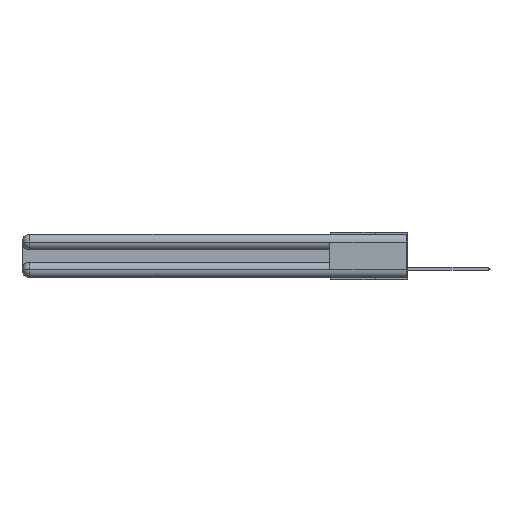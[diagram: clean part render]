
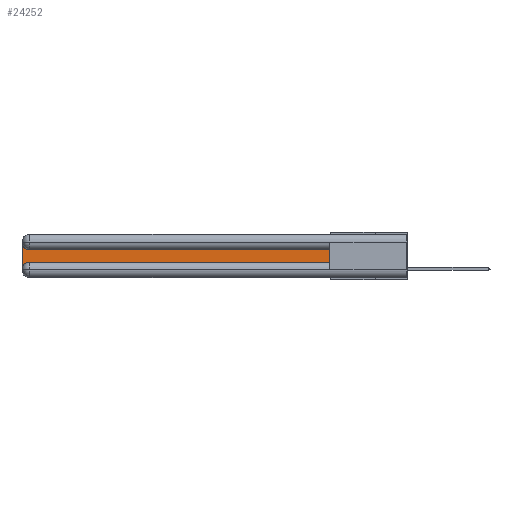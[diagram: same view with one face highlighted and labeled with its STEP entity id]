
A CAD part, left-side view. The second image highlights one B-rep face of the part: STEP entity #24252.
In plain terms, the highlighted planar face has unit normal (-1, 0, 0).
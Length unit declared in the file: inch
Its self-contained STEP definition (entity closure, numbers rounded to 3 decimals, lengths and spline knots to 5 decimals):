
#160 = VERTEX_POINT ( 'NONE', #23383 ) ;
#906 = LINE ( 'NONE', #24101, #9281 ) ;
#1506 = EDGE_CURVE ( 'NONE', #24980, #12879, #25191, .T. ) ;
#2229 = ORIENTED_EDGE ( 'NONE', *, *, #16964, .T. ) ;
#3515 = DIRECTION ( 'NONE',  ( 1., 0., 0. ) ) ;
#4449 = CARTESIAN_POINT ( 'NONE',  ( 0.075, 3., -0.0625 ) ) ;
#4456 = LINE ( 'NONE', #26740, #13216 ) ;
#6352 = LINE ( 'NONE', #27365, #8269 ) ;
#6915 = DIRECTION ( 'NONE',  ( 0., 0., -1. ) ) ;
#7170 = AXIS2_PLACEMENT_3D ( 'NONE', #8288, #17625, #22496 ) ;
#7651 = VECTOR ( 'NONE', #24037, 39.37008 ) ;
#7927 = FACE_OUTER_BOUND ( 'NONE', #24446, .T. ) ;
#7995 = ORIENTED_EDGE ( 'NONE', *, *, #22614, .T. ) ;
#8025 = ORIENTED_EDGE ( 'NONE', *, *, #21451, .T. ) ;
#8269 = VECTOR ( 'NONE', #29788, 39.37008 ) ;
#8288 = CARTESIAN_POINT ( 'NONE',  ( 0.075, 2.94, -0.0625 ) ) ;
#9281 = VECTOR ( 'NONE', #12017, 39.37008 ) ;
#9360 = DIRECTION ( 'NONE',  ( 1., 0., 0. ) ) ;
#9860 = ORIENTED_EDGE ( 'NONE', *, *, #1506, .T. ) ;
#10241 = CARTESIAN_POINT ( 'NONE',  ( 0.075, 0.6, -0.1225 ) ) ;
#10741 = DIRECTION ( 'NONE',  ( 0., 0., -1. ) ) ;
#11388 = EDGE_CURVE ( 'NONE', #23618, #29391, #6352, .T. ) ;
#12017 = DIRECTION ( 'NONE',  ( 0., -1., 0. ) ) ;
#12036 = DIRECTION ( 'NONE',  ( 0., 1., 0. ) ) ;
#12349 = CIRCLE ( 'NONE', #26775, 0.06 ) ;
#12879 = VERTEX_POINT ( 'NONE', #4449 ) ;
#13102 = CARTESIAN_POINT ( 'NONE',  ( 0.075, 3., -0.2775 ) ) ;
#13216 = VECTOR ( 'NONE', #12036, 39.37008 ) ;
#13514 = CARTESIAN_POINT ( 'NONE',  ( 0.075, 2.94, -0.1225 ) ) ;
#15416 = CARTESIAN_POINT ( 'NONE',  ( 0.075, 3., -0.1225 ) ) ;
#16964 = EDGE_CURVE ( 'NONE', #12879, #26027, #19440, .T. ) ;
#17625 = DIRECTION ( 'NONE',  ( 1., 0., 0. ) ) ;
#18729 = CARTESIAN_POINT ( 'NONE',  ( 0.075, 2.94, -0.2775 ) ) ;
#19440 = LINE ( 'NONE', #31328, #7651 ) ;
#21451 = EDGE_CURVE ( 'NONE', #26027, #160, #12349, .T. ) ;
#22496 = DIRECTION ( 'NONE',  ( 0., 0., -1. ) ) ;
#22614 = EDGE_CURVE ( 'NONE', #160, #23618, #906, .T. ) ;
#23040 = PLANE ( 'NONE',  #25805 ) ;
#23383 = CARTESIAN_POINT ( 'NONE',  ( 0.075, 2.94, -0.2175 ) ) ;
#23618 = VERTEX_POINT ( 'NONE', #24094 ) ;
#24037 = DIRECTION ( 'NONE',  ( 0., 0., -1. ) ) ;
#24094 = CARTESIAN_POINT ( 'NONE',  ( 0.075, 0.6, -0.2175 ) ) ;
#24101 = CARTESIAN_POINT ( 'NONE',  ( 0.075, 0.6, -0.2175 ) ) ;
#24252 = ADVANCED_FACE ( 'NONE', ( #7927 ), #23040, .F. ) ;
#24446 = EDGE_LOOP ( 'NONE', ( #25991, #9860, #2229, #8025, #7995, #26131 ) ) ;
#24495 = EDGE_CURVE ( 'NONE', #29391, #24980, #4456, .T. ) ;
#24980 = VERTEX_POINT ( 'NONE', #13514 ) ;
#25191 = CIRCLE ( 'NONE', #7170, 0.06 ) ;
#25805 = AXIS2_PLACEMENT_3D ( 'NONE', #15416, #3515, #10741 ) ;
#25991 = ORIENTED_EDGE ( 'NONE', *, *, #24495, .T. ) ;
#26027 = VERTEX_POINT ( 'NONE', #13102 ) ;
#26131 = ORIENTED_EDGE ( 'NONE', *, *, #11388, .T. ) ;
#26740 = CARTESIAN_POINT ( 'NONE',  ( 0.075, 0.6, -0.1225 ) ) ;
#26775 = AXIS2_PLACEMENT_3D ( 'NONE', #18729, #9360, #6915 ) ;
#27365 = CARTESIAN_POINT ( 'NONE',  ( 0.075, 0.6, -0.2175 ) ) ;
#29391 = VERTEX_POINT ( 'NONE', #10241 ) ;
#29788 = DIRECTION ( 'NONE',  ( 0., 0., 1. ) ) ;
#31328 = CARTESIAN_POINT ( 'NONE',  ( 0.075, 3., -0.2175 ) ) ;
